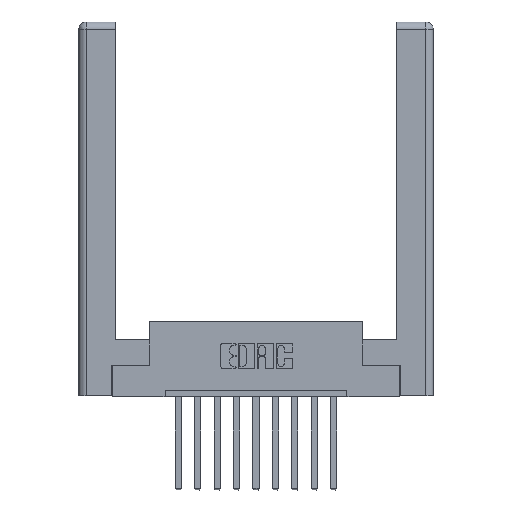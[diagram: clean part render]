
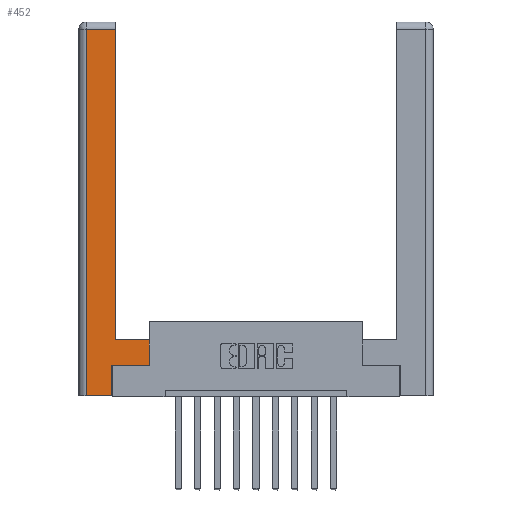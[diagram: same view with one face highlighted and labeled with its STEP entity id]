
A CAD part, top view. The second image highlights one B-rep face of the part: STEP entity #452.
In plain terms, the highlighted planar face has unit normal (0, 0, 1).
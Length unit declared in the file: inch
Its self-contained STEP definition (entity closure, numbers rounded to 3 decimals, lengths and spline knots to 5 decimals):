
#71 = DIRECTION ( 'NONE',  ( 1., 0., 0. ) ) ;
#452 = ADVANCED_FACE ( 'NONE', ( #9798 ), #4009, .F. ) ;
#882 = CARTESIAN_POINT ( 'NONE',  ( 0.0615, 2.94, 0. ) ) ;
#930 = CARTESIAN_POINT ( 'NONE',  ( 0., 0., 0. ) ) ;
#1116 = LINE ( 'NONE', #4432, #12470 ) ;
#1202 = CARTESIAN_POINT ( 'NONE',  ( 0.295, 3., 0. ) ) ;
#1315 = VECTOR ( 'NONE', #8549, 39.37008 ) ;
#1415 = EDGE_CURVE ( 'NONE', #6567, #1574, #9935, .T. ) ;
#1574 = VERTEX_POINT ( 'NONE', #13087 ) ;
#1657 = VERTEX_POINT ( 'NONE', #8634 ) ;
#2565 = VERTEX_POINT ( 'NONE', #7226 ) ;
#2643 = VERTEX_POINT ( 'NONE', #12559 ) ;
#2789 = CARTESIAN_POINT ( 'NONE',  ( 0.0615, 0., 0. ) ) ;
#3274 = EDGE_CURVE ( 'NONE', #2643, #1657, #6309, .T. ) ;
#3428 = CARTESIAN_POINT ( 'NONE',  ( 0.0615, 2.94, 0. ) ) ;
#3451 = EDGE_CURVE ( 'NONE', #8900, #2643, #1116, .T. ) ;
#3464 = ORIENTED_EDGE ( 'NONE', *, *, #7694, .T. ) ;
#4009 = PLANE ( 'NONE',  #4012 ) ;
#4012 = AXIS2_PLACEMENT_3D ( 'NONE', #930, #6138, #5097 ) ;
#4348 = EDGE_CURVE ( 'NONE', #12486, #2565, #12289, .T. ) ;
#4432 = CARTESIAN_POINT ( 'NONE',  ( 0.265, 0.245, 0. ) ) ;
#4473 = CARTESIAN_POINT ( 'NONE',  ( 0.565, 0.45, 0. ) ) ;
#4842 = CARTESIAN_POINT ( 'NONE',  ( 0.265, 0., 0. ) ) ;
#5043 = DIRECTION ( 'NONE',  ( -1., 0., 0. ) ) ;
#5080 = CARTESIAN_POINT ( 'NONE',  ( 0.565, 0.45, 0. ) ) ;
#5097 = DIRECTION ( 'NONE',  ( -1., 0., 0. ) ) ;
#5155 = EDGE_CURVE ( 'NONE', #1657, #7007, #9507, .T. ) ;
#5156 = VECTOR ( 'NONE', #13137, 39.37008 ) ;
#5317 = CARTESIAN_POINT ( 'NONE',  ( 0.295, 0.45, 0. ) ) ;
#5588 = DIRECTION ( 'NONE',  ( -1., 0., 0. ) ) ;
#5624 = CARTESIAN_POINT ( 'NONE',  ( 0.295, 0.45, 0. ) ) ;
#5660 = DIRECTION ( 'NONE',  ( 0., 1., 0. ) ) ;
#6138 = DIRECTION ( 'NONE',  ( 0., 0., -1. ) ) ;
#6219 = EDGE_CURVE ( 'NONE', #1574, #12486, #6241, .T. ) ;
#6241 = LINE ( 'NONE', #882, #10783 ) ;
#6309 = LINE ( 'NONE', #10383, #10377 ) ;
#6567 = VERTEX_POINT ( 'NONE', #5624 ) ;
#7007 = VERTEX_POINT ( 'NONE', #4473 ) ;
#7226 = CARTESIAN_POINT ( 'NONE',  ( 0.0615, 0., 0. ) ) ;
#7694 = EDGE_CURVE ( 'NONE', #7007, #6567, #12357, .T. ) ;
#8190 = ORIENTED_EDGE ( 'NONE', *, *, #4348, .T. ) ;
#8549 = DIRECTION ( 'NONE',  ( 0., 1., 0. ) ) ;
#8634 = CARTESIAN_POINT ( 'NONE',  ( 0.565, 0.245, 0. ) ) ;
#8897 = CARTESIAN_POINT ( 'NONE',  ( 0.265, 0., 0. ) ) ;
#8900 = VERTEX_POINT ( 'NONE', #4842 ) ;
#9161 = VECTOR ( 'NONE', #11994, 39.37008 ) ;
#9194 = VECTOR ( 'NONE', #11330, 39.37008 ) ;
#9507 = LINE ( 'NONE', #5080, #9194 ) ;
#9532 = EDGE_CURVE ( 'NONE', #2565, #8900, #10603, .T. ) ;
#9798 = FACE_OUTER_BOUND ( 'NONE', #12149, .T. ) ;
#9935 = LINE ( 'NONE', #1202, #1315 ) ;
#9978 = ORIENTED_EDGE ( 'NONE', *, *, #6219, .T. ) ;
#10377 = VECTOR ( 'NONE', #71, 39.37008 ) ;
#10383 = CARTESIAN_POINT ( 'NONE',  ( 0.565, 0.245, 0. ) ) ;
#10603 = LINE ( 'NONE', #8897, #9161 ) ;
#10783 = VECTOR ( 'NONE', #5043, 39.37008 ) ;
#10922 = ORIENTED_EDGE ( 'NONE', *, *, #9532, .T. ) ;
#11330 = DIRECTION ( 'NONE',  ( 0., 1., 0. ) ) ;
#11540 = ORIENTED_EDGE ( 'NONE', *, *, #3451, .T. ) ;
#11994 = DIRECTION ( 'NONE',  ( 1., 0., 0. ) ) ;
#12149 = EDGE_LOOP ( 'NONE', ( #12203, #9978, #8190, #10922, #11540, #13354, #12245, #3464 ) ) ;
#12203 = ORIENTED_EDGE ( 'NONE', *, *, #1415, .T. ) ;
#12207 = VECTOR ( 'NONE', #5588, 39.37008 ) ;
#12245 = ORIENTED_EDGE ( 'NONE', *, *, #5155, .T. ) ;
#12289 = LINE ( 'NONE', #2789, #5156 ) ;
#12357 = LINE ( 'NONE', #5317, #12207 ) ;
#12470 = VECTOR ( 'NONE', #5660, 39.37008 ) ;
#12486 = VERTEX_POINT ( 'NONE', #3428 ) ;
#12559 = CARTESIAN_POINT ( 'NONE',  ( 0.265, 0.245, 0. ) ) ;
#13087 = CARTESIAN_POINT ( 'NONE',  ( 0.295, 2.94, 0. ) ) ;
#13137 = DIRECTION ( 'NONE',  ( 0., -1., 0. ) ) ;
#13354 = ORIENTED_EDGE ( 'NONE', *, *, #3274, .T. ) ;
